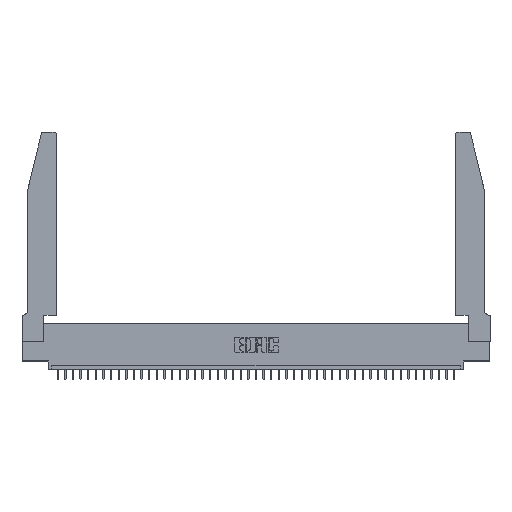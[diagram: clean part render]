
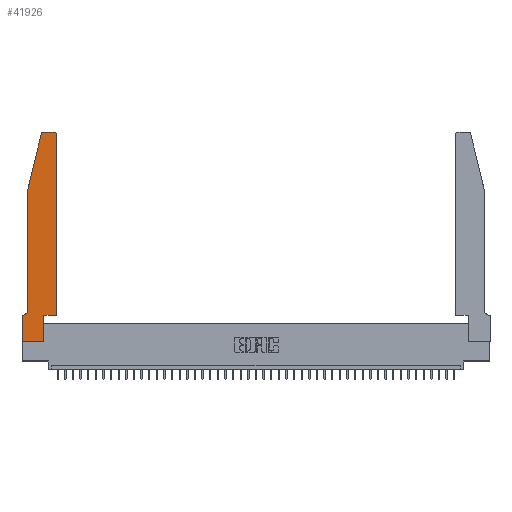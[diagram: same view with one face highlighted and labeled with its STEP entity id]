
A CAD part, top view. The second image highlights one B-rep face of the part: STEP entity #41926.
In plain terms, the highlighted planar face has unit normal (0, 0, 1).
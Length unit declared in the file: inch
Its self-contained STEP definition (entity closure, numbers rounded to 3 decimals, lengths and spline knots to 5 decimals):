
#98 = CARTESIAN_POINT ( 'NONE',  ( 0.4505, 0.35, 0.37 ) ) ;
#288 = CARTESIAN_POINT ( 'NONE',  ( 0., 0., 0.37 ) ) ;
#361 = DIRECTION ( 'NONE',  ( 0., -1., 0. ) ) ;
#1494 = DIRECTION ( 'NONE',  ( 0., -1., 0. ) ) ;
#2950 = CARTESIAN_POINT ( 'NONE',  ( 0., 0., 0.37 ) ) ;
#3819 = EDGE_CURVE ( 'NONE', #34012, #18071, #10795, .T. ) ;
#4274 = EDGE_CURVE ( 'NONE', #37064, #21785, #39153, .T. ) ;
#4591 = DIRECTION ( 'NONE',  ( 0., 0., 1. ) ) ;
#4889 = ORIENTED_EDGE ( 'NONE', *, *, #4274, .T. ) ;
#5192 = EDGE_CURVE ( 'NONE', #21785, #43138, #9370, .T. ) ;
#5422 = DIRECTION ( 'NONE',  ( -1., 0., 0. ) ) ;
#6686 = ORIENTED_EDGE ( 'NONE', *, *, #17229, .T. ) ;
#6715 = DIRECTION ( 'NONE',  ( 0., 1., 0. ) ) ;
#6973 = VERTEX_POINT ( 'NONE', #20927 ) ;
#7496 = CARTESIAN_POINT ( 'NONE',  ( 0.2605, 2.75, 0.37 ) ) ;
#7540 = FACE_OUTER_BOUND ( 'NONE', #19407, .T. ) ;
#8486 = AXIS2_PLACEMENT_3D ( 'NONE', #28910, #4591, #25606 ) ;
#8780 = AXIS2_PLACEMENT_3D ( 'NONE', #23760, #13899, #27289 ) ;
#9138 = CARTESIAN_POINT ( 'NONE',  ( 0.0755, 0.35, 0.37 ) ) ;
#9370 = LINE ( 'NONE', #23180, #26735 ) ;
#9433 = CARTESIAN_POINT ( 'NONE',  ( 0.4505, 2.72, 0.37 ) ) ;
#9849 = EDGE_CURVE ( 'NONE', #36153, #18004, #10117, .T. ) ;
#10028 = CIRCLE ( 'NONE', #11414, 0.07 ) ;
#10117 = LINE ( 'NONE', #23479, #17052 ) ;
#10795 = LINE ( 'NONE', #7496, #16835 ) ;
#11414 = AXIS2_PLACEMENT_3D ( 'NONE', #37883, #11583, #5422 ) ;
#11575 = CARTESIAN_POINT ( 'NONE',  ( 0.2865, 0.35, 0.37 ) ) ;
#11583 = DIRECTION ( 'NONE',  ( 0., 0., -1. ) ) ;
#12306 = CARTESIAN_POINT ( 'NONE',  ( 0.0055, 0.35, 0.37 ) ) ;
#12430 = VECTOR ( 'NONE', #1494, 39.37008 ) ;
#12462 = ORIENTED_EDGE ( 'NONE', *, *, #36253, .T. ) ;
#12744 = CARTESIAN_POINT ( 'NONE',  ( 0.25487, 2.72718, 0.37 ) ) ;
#13010 = ORIENTED_EDGE ( 'NONE', *, *, #5192, .T. ) ;
#13899 = DIRECTION ( 'NONE',  ( 0., 0., 1. ) ) ;
#14475 = DIRECTION ( 'NONE',  ( 1., 0., 0. ) ) ;
#15269 = EDGE_CURVE ( 'NONE', #43138, #23444, #43319, .T. ) ;
#15282 = VECTOR ( 'NONE', #30014, 39.37008 ) ;
#15619 = ORIENTED_EDGE ( 'NONE', *, *, #15269, .T. ) ;
#15847 = ORIENTED_EDGE ( 'NONE', *, *, #38127, .T. ) ;
#16119 = DIRECTION ( 'NONE',  ( -1., 0., 0. ) ) ;
#16353 = EDGE_CURVE ( 'NONE', #41492, #6973, #38114, .T. ) ;
#16625 = CARTESIAN_POINT ( 'NONE',  ( 0.4205, 2.75, 0.37 ) ) ;
#16811 = LINE ( 'NONE', #30665, #15282 ) ;
#16835 = VECTOR ( 'NONE', #24133, 39.37008 ) ;
#17052 = VECTOR ( 'NONE', #14475, 39.37008 ) ;
#17229 = EDGE_CURVE ( 'NONE', #40111, #41492, #16811, .T. ) ;
#18004 = VERTEX_POINT ( 'NONE', #37777 ) ;
#18037 = CIRCLE ( 'NONE', #20852, 0.03 ) ;
#18071 = VERTEX_POINT ( 'NONE', #21109 ) ;
#18300 = EDGE_CURVE ( 'NONE', #18071, #40111, #18037, .T. ) ;
#18955 = VECTOR ( 'NONE', #16119, 39.37008 ) ;
#19100 = VECTOR ( 'NONE', #27827, 39.37008 ) ;
#19407 = EDGE_LOOP ( 'NONE', ( #29555, #33206, #6686, #41237, #30940, #4889, #13010, #15619, #39694, #33591, #15847, #12462 ) ) ;
#19835 = CARTESIAN_POINT ( 'NONE',  ( 0.2865, 0.35, 0.37 ) ) ;
#20224 = CARTESIAN_POINT ( 'NONE',  ( 0., 0.35, 0.37 ) ) ;
#20852 = AXIS2_PLACEMENT_3D ( 'NONE', #39259, #43018, #39696 ) ;
#20927 = CARTESIAN_POINT ( 'NONE',  ( 0.0755, 0.42, 0.37 ) ) ;
#21109 = CARTESIAN_POINT ( 'NONE',  ( 0.284, 2.75, 0.37 ) ) ;
#21785 = VERTEX_POINT ( 'NONE', #20224 ) ;
#22065 = LINE ( 'NONE', #11575, #19100 ) ;
#23134 = DIRECTION ( 'NONE',  ( 1., 0., 0. ) ) ;
#23180 = CARTESIAN_POINT ( 'NONE',  ( 0., 0., 0.37 ) ) ;
#23444 = VERTEX_POINT ( 'NONE', #34126 ) ;
#23479 = CARTESIAN_POINT ( 'NONE',  ( 0.4505, 0.35, 0.37 ) ) ;
#23760 = CARTESIAN_POINT ( 'NONE',  ( 0., 0.35, 0.37 ) ) ;
#24024 = CARTESIAN_POINT ( 'NONE',  ( 0.0755, 2., 0.37 ) ) ;
#24133 = DIRECTION ( 'NONE',  ( -1., 0., 0. ) ) ;
#25606 = DIRECTION ( 'NONE',  ( 1., 0., 0. ) ) ;
#26735 = VECTOR ( 'NONE', #361, 39.37008 ) ;
#26766 = VECTOR ( 'NONE', #6715, 39.37008 ) ;
#27073 = VERTEX_POINT ( 'NONE', #9433 ) ;
#27289 = DIRECTION ( 'NONE',  ( 1., 0., 0. ) ) ;
#27827 = DIRECTION ( 'NONE',  ( 0., 1., 0. ) ) ;
#28680 = EDGE_CURVE ( 'NONE', #23444, #36153, #22065, .T. ) ;
#28910 = CARTESIAN_POINT ( 'NONE',  ( 0.4205, 2.72, 0.37 ) ) ;
#29555 = ORIENTED_EDGE ( 'NONE', *, *, #3819, .T. ) ;
#30014 = DIRECTION ( 'NONE',  ( -0.239, -0.971, 0. ) ) ;
#30067 = EDGE_CURVE ( 'NONE', #6973, #37064, #10028, .T. ) ;
#30665 = CARTESIAN_POINT ( 'NONE',  ( 0.0755, 2., 0.37 ) ) ;
#30940 = ORIENTED_EDGE ( 'NONE', *, *, #30067, .T. ) ;
#33206 = ORIENTED_EDGE ( 'NONE', *, *, #18300, .T. ) ;
#33356 = VECTOR ( 'NONE', #23134, 39.37008 ) ;
#33591 = ORIENTED_EDGE ( 'NONE', *, *, #9849, .T. ) ;
#34012 = VERTEX_POINT ( 'NONE', #16625 ) ;
#34126 = CARTESIAN_POINT ( 'NONE',  ( 0.2865, 0., 0.37 ) ) ;
#34294 = LINE ( 'NONE', #98, #26766 ) ;
#36153 = VERTEX_POINT ( 'NONE', #19835 ) ;
#36253 = EDGE_CURVE ( 'NONE', #27073, #34012, #42782, .T. ) ;
#37064 = VERTEX_POINT ( 'NONE', #12306 ) ;
#37555 = PLANE ( 'NONE',  #8780 ) ;
#37777 = CARTESIAN_POINT ( 'NONE',  ( 0.4505, 0.35, 0.37 ) ) ;
#37883 = CARTESIAN_POINT ( 'NONE',  ( 0.0055, 0.42, 0.37 ) ) ;
#38114 = LINE ( 'NONE', #41402, #12430 ) ;
#38127 = EDGE_CURVE ( 'NONE', #18004, #27073, #34294, .T. ) ;
#39153 = LINE ( 'NONE', #9138, #18955 ) ;
#39259 = CARTESIAN_POINT ( 'NONE',  ( 0.284, 2.72, 0.37 ) ) ;
#39694 = ORIENTED_EDGE ( 'NONE', *, *, #28680, .T. ) ;
#39696 = DIRECTION ( 'NONE',  ( 1., 0., 0. ) ) ;
#40111 = VERTEX_POINT ( 'NONE', #12744 ) ;
#41237 = ORIENTED_EDGE ( 'NONE', *, *, #16353, .T. ) ;
#41402 = CARTESIAN_POINT ( 'NONE',  ( 0.0755, 2., 0.37 ) ) ;
#41492 = VERTEX_POINT ( 'NONE', #24024 ) ;
#41926 = ADVANCED_FACE ( 'NONE', ( #7540 ), #37555, .T. ) ;
#42782 = CIRCLE ( 'NONE', #8486, 0.03 ) ;
#43018 = DIRECTION ( 'NONE',  ( 0., 0., 1. ) ) ;
#43138 = VERTEX_POINT ( 'NONE', #288 ) ;
#43319 = LINE ( 'NONE', #2950, #33356 ) ;
